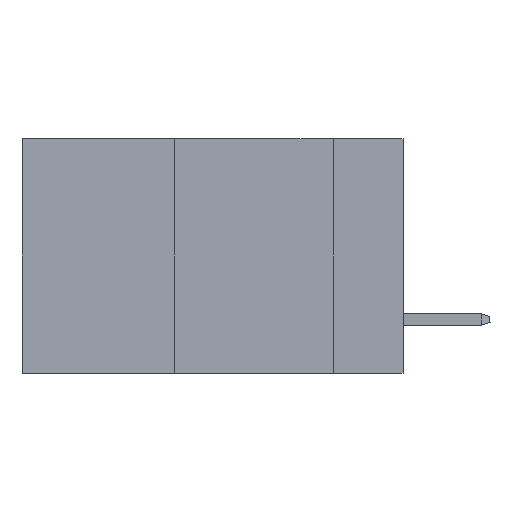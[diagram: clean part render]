
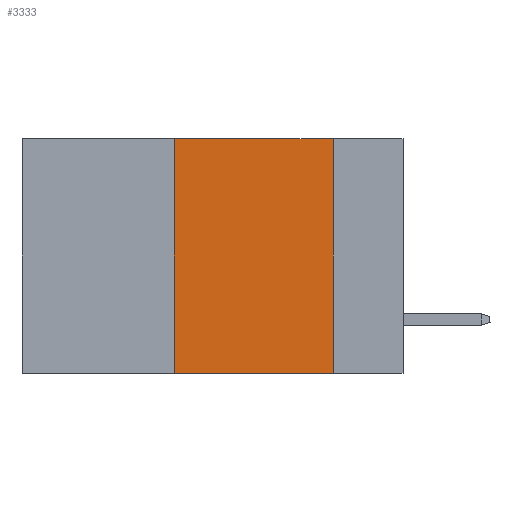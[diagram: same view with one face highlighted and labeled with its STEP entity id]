
A CAD part, left-side view. The second image highlights one B-rep face of the part: STEP entity #3333.
In plain terms, the highlighted planar face has unit normal (-1, 0, 0).
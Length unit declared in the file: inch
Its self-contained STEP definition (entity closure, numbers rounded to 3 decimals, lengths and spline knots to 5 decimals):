
#208 = ORIENTED_EDGE ( 'NONE', *, *, #25785, .T. ) ;
#662 = LINE ( 'NONE', #9124, #1552 ) ;
#727 = VERTEX_POINT ( 'NONE', #2377 ) ;
#1165 = CARTESIAN_POINT ( 'NONE',  ( 0., 0.11, -0.37 ) ) ;
#1552 = VECTOR ( 'NONE', #26368, 39.37008 ) ;
#1689 = DIRECTION ( 'NONE',  ( 0., 0., -1. ) ) ;
#2377 = CARTESIAN_POINT ( 'NONE',  ( 0., 0.36, -0.37 ) ) ;
#3333 = ADVANCED_FACE ( 'NONE', ( #5865 ), #11821, .F. ) ;
#4166 = LINE ( 'NONE', #5848, #23990 ) ;
#4412 = EDGE_LOOP ( 'NONE', ( #20537, #17963, #10344, #208 ) ) ;
#5848 = CARTESIAN_POINT ( 'NONE',  ( 0., 0.11, 0. ) ) ;
#5865 = FACE_OUTER_BOUND ( 'NONE', #4412, .T. ) ;
#8490 = VERTEX_POINT ( 'NONE', #13568 ) ;
#9124 = CARTESIAN_POINT ( 'NONE',  ( 0., 0.6, -0.37 ) ) ;
#10344 = ORIENTED_EDGE ( 'NONE', *, *, #25697, .F. ) ;
#10772 = LINE ( 'NONE', #19260, #13008 ) ;
#11254 = DIRECTION ( 'NONE',  ( 0., -1., 0. ) ) ;
#11687 = CARTESIAN_POINT ( 'NONE',  ( 0., 0.6, 0. ) ) ;
#11821 = PLANE ( 'NONE',  #19695 ) ;
#12904 = CARTESIAN_POINT ( 'NONE',  ( 0., 0.36, 0. ) ) ;
#13008 = VECTOR ( 'NONE', #14799, 39.37008 ) ;
#13265 = VERTEX_POINT ( 'NONE', #12904 ) ;
#13341 = CARTESIAN_POINT ( 'NONE',  ( 0., 0.6, 0. ) ) ;
#13568 = CARTESIAN_POINT ( 'NONE',  ( 0., 0.11, 0. ) ) ;
#14799 = DIRECTION ( 'NONE',  ( 0., 0., 1. ) ) ;
#15855 = DIRECTION ( 'NONE',  ( 1., 0., 0. ) ) ;
#17963 = ORIENTED_EDGE ( 'NONE', *, *, #19429, .F. ) ;
#18444 = VERTEX_POINT ( 'NONE', #1165 ) ;
#19046 = VECTOR ( 'NONE', #11254, 39.37008 ) ;
#19260 = CARTESIAN_POINT ( 'NONE',  ( 0., 0.36, 0. ) ) ;
#19429 = EDGE_CURVE ( 'NONE', #13265, #8490, #19608, .T. ) ;
#19608 = LINE ( 'NONE', #13341, #19046 ) ;
#19620 = EDGE_CURVE ( 'NONE', #8490, #18444, #4166, .T. ) ;
#19695 = AXIS2_PLACEMENT_3D ( 'NONE', #11687, #15855, #24373 ) ;
#20537 = ORIENTED_EDGE ( 'NONE', *, *, #19620, .F. ) ;
#23990 = VECTOR ( 'NONE', #1689, 39.37008 ) ;
#24373 = DIRECTION ( 'NONE',  ( 0., 0., -1. ) ) ;
#25697 = EDGE_CURVE ( 'NONE', #727, #13265, #10772, .T. ) ;
#25785 = EDGE_CURVE ( 'NONE', #727, #18444, #662, .T. ) ;
#26368 = DIRECTION ( 'NONE',  ( 0., -1., 0. ) ) ;
